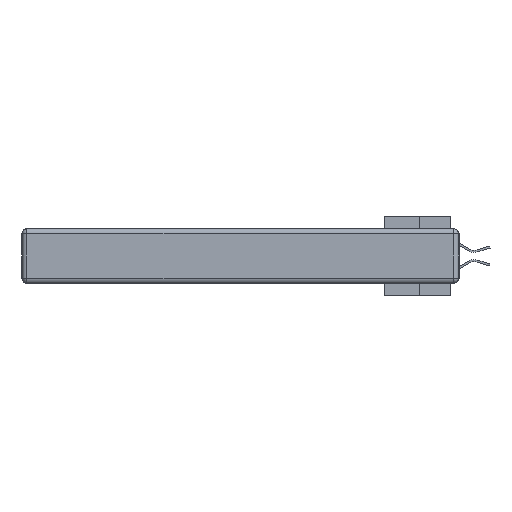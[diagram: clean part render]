
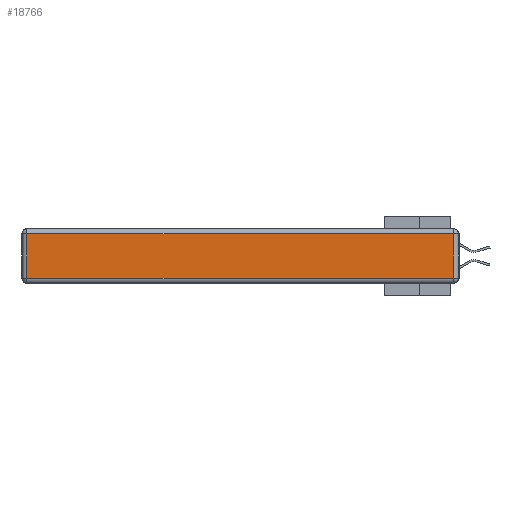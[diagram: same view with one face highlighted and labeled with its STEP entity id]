
A CAD part, left-side view. The second image highlights one B-rep face of the part: STEP entity #18766.
In plain terms, the highlighted planar face has unit normal (-1, 0, 0).
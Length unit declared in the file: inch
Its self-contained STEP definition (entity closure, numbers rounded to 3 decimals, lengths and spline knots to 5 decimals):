
#351 = PLANE ( 'NONE',  #21493 ) ;
#4121 = VECTOR ( 'NONE', #12023, 39.37008 ) ;
#5396 = VERTEX_POINT ( 'NONE', #29867 ) ;
#6555 = ORIENTED_EDGE ( 'NONE', *, *, #28485, .T. ) ;
#7358 = CARTESIAN_POINT ( 'NONE',  ( 0., 2.72, -0.03 ) ) ;
#7881 = ORIENTED_EDGE ( 'NONE', *, *, #14898, .T. ) ;
#8705 = DIRECTION ( 'NONE',  ( 0., 0., 1. ) ) ;
#9204 = DIRECTION ( 'NONE',  ( 0., 0., 1. ) ) ;
#9399 = CARTESIAN_POINT ( 'NONE',  ( 0., 0., -0.313 ) ) ;
#9572 = VERTEX_POINT ( 'NONE', #20133 ) ;
#9843 = CARTESIAN_POINT ( 'NONE',  ( 0., 2.75, -0.03 ) ) ;
#11306 = CARTESIAN_POINT ( 'NONE',  ( 0., 2.72, -0.343 ) ) ;
#11856 = CARTESIAN_POINT ( 'NONE',  ( 0., 0., -0.343 ) ) ;
#12023 = DIRECTION ( 'NONE',  ( 0., -1., 0. ) ) ;
#13436 = LINE ( 'NONE', #9843, #35437 ) ;
#13556 = LINE ( 'NONE', #9399, #4121 ) ;
#14898 = EDGE_CURVE ( 'NONE', #22991, #35263, #13436, .T. ) ;
#18145 = EDGE_CURVE ( 'NONE', #9572, #22991, #26223, .T. ) ;
#18158 = CARTESIAN_POINT ( 'NONE',  ( 0., 0.03, -0.343 ) ) ;
#18766 = ADVANCED_FACE ( 'NONE', ( #31141 ), #351, .T. ) ;
#20133 = CARTESIAN_POINT ( 'NONE',  ( 0., 0.03, -0.313 ) ) ;
#20311 = ORIENTED_EDGE ( 'NONE', *, *, #35143, .T. ) ;
#21419 = LINE ( 'NONE', #11306, #25435 ) ;
#21493 = AXIS2_PLACEMENT_3D ( 'NONE', #11856, #35093, #8705 ) ;
#22991 = VERTEX_POINT ( 'NONE', #26569 ) ;
#23316 = EDGE_LOOP ( 'NONE', ( #20311, #24656, #7881, #6555 ) ) ;
#24656 = ORIENTED_EDGE ( 'NONE', *, *, #18145, .T. ) ;
#25435 = VECTOR ( 'NONE', #34675, 39.37008 ) ;
#26223 = LINE ( 'NONE', #18158, #31135 ) ;
#26569 = CARTESIAN_POINT ( 'NONE',  ( 0., 0.03, -0.03 ) ) ;
#28485 = EDGE_CURVE ( 'NONE', #35263, #5396, #21419, .T. ) ;
#29867 = CARTESIAN_POINT ( 'NONE',  ( 0., 2.72, -0.313 ) ) ;
#31135 = VECTOR ( 'NONE', #9204, 39.37008 ) ;
#31141 = FACE_OUTER_BOUND ( 'NONE', #23316, .T. ) ;
#32851 = DIRECTION ( 'NONE',  ( 0., 1., 0. ) ) ;
#34675 = DIRECTION ( 'NONE',  ( 0., 0., -1. ) ) ;
#35093 = DIRECTION ( 'NONE',  ( -1., 0., 0. ) ) ;
#35143 = EDGE_CURVE ( 'NONE', #5396, #9572, #13556, .T. ) ;
#35263 = VERTEX_POINT ( 'NONE', #7358 ) ;
#35437 = VECTOR ( 'NONE', #32851, 39.37008 ) ;
